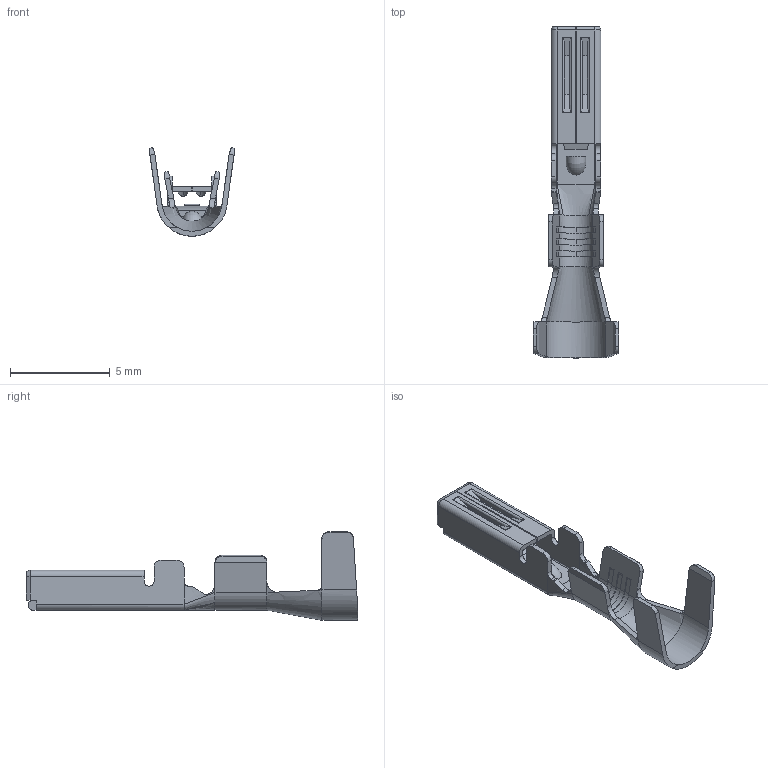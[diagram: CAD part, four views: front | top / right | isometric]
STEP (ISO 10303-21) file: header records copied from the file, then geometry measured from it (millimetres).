
FILE_DESCRIPTION (( 'STEP AP214' ), '1' );
FILE_NAME ('570-290-721.STEP', '2020-09-17T19:58:52', ( '' ), ( '' ), 'SwSTEP 2.0', 'SolidWorks 2020', '' );
FILE_SCHEMA (( 'AUTOMOTIVE_DESIGN' ));
Length unit declared in the file: millimetre
Products named in the file (1): 570-290-721
Bounding box: 4.3 x 16.6 x 4.42 mm (x, y, z)
Volume: 28.6 mm3; surface area: 258 mm2
Topology: 1 solids, 1 shells, 242 faces, 641 edges, 409 vertices
Faces by surface type: plane 111, cylinder 98, bspline 27, cone 4, torus 2
Entity records: 8876 total; most frequent: CARTESIAN_POINT 3165, ORIENTED_EDGE 1282, DIRECTION 1026, EDGE_CURVE 641, VERTEX_POINT 409, VECTOR 364, LINE 364, AXIS2_PLACEMENT_3D 331
